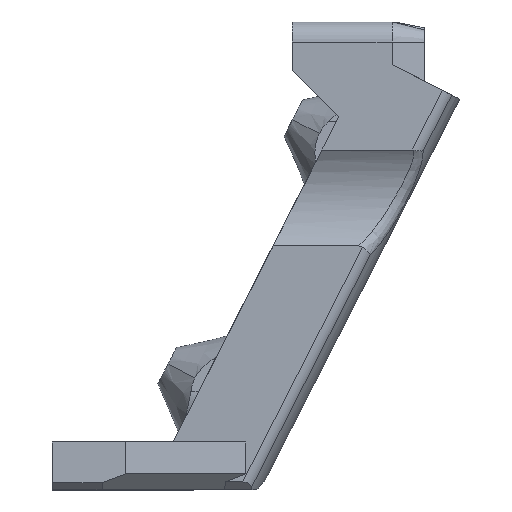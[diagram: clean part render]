
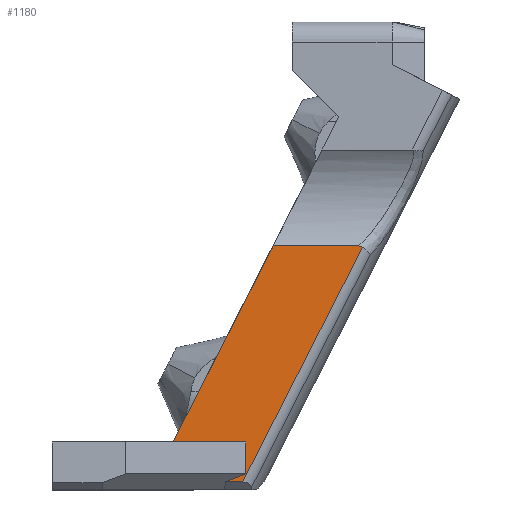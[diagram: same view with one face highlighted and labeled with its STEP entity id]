
A CAD part, front view. The second image highlights one B-rep face of the part: STEP entity #1180.
In plain terms, the highlighted planar face has unit normal (0, -1, 0).
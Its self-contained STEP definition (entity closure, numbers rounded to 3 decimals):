
#31=B_SPLINE_CURVE_WITH_KNOTS('',3,(#1776,#1777,#1778,#1779,#1780,#1781,
#1782,#1783,#1784,#1785,#1786,#1787,#1788,#1789,#1790,#1791),
 .UNSPECIFIED.,.F.,.F.,(4,3,3,3,3,4),(0.,0.009,0.017,
0.017,0.025,0.031),.UNSPECIFIED.);
#116=FACE_OUTER_BOUND('',#183,.T.);
#183=EDGE_LOOP('',(#814,#815,#816,#817,#818,#819,#820,#821));
#266=LINE('',#1768,#377);
#269=LINE('',#1774,#380);
#270=LINE('',#1793,#381);
#271=LINE('',#1795,#382);
#272=LINE('',#1797,#383);
#273=LINE('',#1799,#384);
#274=LINE('',#1800,#385);
#377=VECTOR('',#1420,10.);
#380=VECTOR('',#1425,10.);
#381=VECTOR('',#1426,10.);
#382=VECTOR('',#1427,10.);
#383=VECTOR('',#1428,10.);
#384=VECTOR('',#1429,10.);
#385=VECTOR('',#1430,10.);
#498=VERTEX_POINT('',#1765);
#499=VERTEX_POINT('',#1767);
#501=VERTEX_POINT('',#1773);
#502=VERTEX_POINT('',#1775);
#503=VERTEX_POINT('',#1792);
#504=VERTEX_POINT('',#1794);
#505=VERTEX_POINT('',#1796);
#506=VERTEX_POINT('',#1798);
#622=EDGE_CURVE('',#498,#499,#266,.T.);
#625=EDGE_CURVE('',#501,#498,#269,.T.);
#626=EDGE_CURVE('',#502,#501,#31,.T.);
#627=EDGE_CURVE('',#503,#502,#270,.T.);
#628=EDGE_CURVE('',#503,#504,#271,.T.);
#629=EDGE_CURVE('',#504,#505,#272,.T.);
#630=EDGE_CURVE('',#505,#506,#273,.T.);
#631=EDGE_CURVE('',#499,#506,#274,.F.);
#814=ORIENTED_EDGE('',*,*,#622,.F.);
#815=ORIENTED_EDGE('',*,*,#625,.F.);
#816=ORIENTED_EDGE('',*,*,#626,.F.);
#817=ORIENTED_EDGE('',*,*,#627,.F.);
#818=ORIENTED_EDGE('',*,*,#628,.T.);
#819=ORIENTED_EDGE('',*,*,#629,.T.);
#820=ORIENTED_EDGE('',*,*,#630,.T.);
#821=ORIENTED_EDGE('',*,*,#631,.F.);
#1133=PLANE('',#1274);
#1180=ADVANCED_FACE('',(#116),#1133,.T.);
#1274=AXIS2_PLACEMENT_3D('',#1772,#1423,#1424);
#1420=DIRECTION('',(-1.,0.,0.));
#1423=DIRECTION('center_axis',(0.,-1.,0.));
#1424=DIRECTION('ref_axis',(0.,0.,-1.));
#1425=DIRECTION('',(-0.454,0.,-0.891));
#1426=DIRECTION('',(1.,0.,0.));
#1427=DIRECTION('',(-0.454,0.,-0.891));
#1428=DIRECTION('',(1.,0.,0.));
#1429=DIRECTION('',(0.,0.,-1.));
#1430=DIRECTION('',(-0.929,0.,-0.37));
#1765=CARTESIAN_POINT('',(14.449,-14.625,0.5));
#1767=CARTESIAN_POINT('',(13.392,-14.625,0.5));
#1768=CARTESIAN_POINT('',(5.55,-14.625,0.5));
#1772=CARTESIAN_POINT('Origin',(5.55,-14.625,29.25));
#1773=CARTESIAN_POINT('',(21.925,-14.625,15.171));
#1774=CARTESIAN_POINT('',(26.718,-14.625,24.579));
#1775=CARTESIAN_POINT('',(21.631,-14.625,15.25));
#1776=CARTESIAN_POINT('Ctrl Pts',(21.631,-14.625,15.25));
#1777=CARTESIAN_POINT('Ctrl Pts',(21.66,-14.625,15.25));
#1778=CARTESIAN_POINT('Ctrl Pts',(21.689,-14.625,15.248));
#1779=CARTESIAN_POINT('Ctrl Pts',(21.717,-14.625,15.245));
#1780=CARTESIAN_POINT('Ctrl Pts',(21.744,-14.625,15.242));
#1781=CARTESIAN_POINT('Ctrl Pts',(21.771,-14.625,15.237));
#1782=CARTESIAN_POINT('Ctrl Pts',(21.797,-14.625,15.23));
#1783=CARTESIAN_POINT('Ctrl Pts',(21.798,-14.625,15.229));
#1784=CARTESIAN_POINT('Ctrl Pts',(21.8,-14.625,15.229));
#1785=CARTESIAN_POINT('Ctrl Pts',(21.802,-14.625,15.228));
#1786=CARTESIAN_POINT('Ctrl Pts',(21.826,-14.625,15.221));
#1787=CARTESIAN_POINT('Ctrl Pts',(21.85,-14.625,15.212));
#1788=CARTESIAN_POINT('Ctrl Pts',(21.873,-14.625,15.201));
#1789=CARTESIAN_POINT('Ctrl Pts',(21.891,-14.625,15.192));
#1790=CARTESIAN_POINT('Ctrl Pts',(21.908,-14.625,15.182));
#1791=CARTESIAN_POINT('Ctrl Pts',(21.924,-14.625,15.17));
#1792=CARTESIAN_POINT('',(16.339,-14.625,15.25));
#1793=CARTESIAN_POINT('',(5.55,-14.625,15.25));
#1794=CARTESIAN_POINT('',(10.097,-14.625,3.));
#1795=CARTESIAN_POINT('',(14.938,-14.625,12.5));
#1796=CARTESIAN_POINT('',(14.646,-14.625,3.));
#1797=CARTESIAN_POINT('',(7.824,-14.625,3.));
#1798=CARTESIAN_POINT('',(14.646,-14.625,1.));
#1799=CARTESIAN_POINT('',(14.646,-14.625,14.625));
#1800=CARTESIAN_POINT('',(12.137,-14.625,0.));
